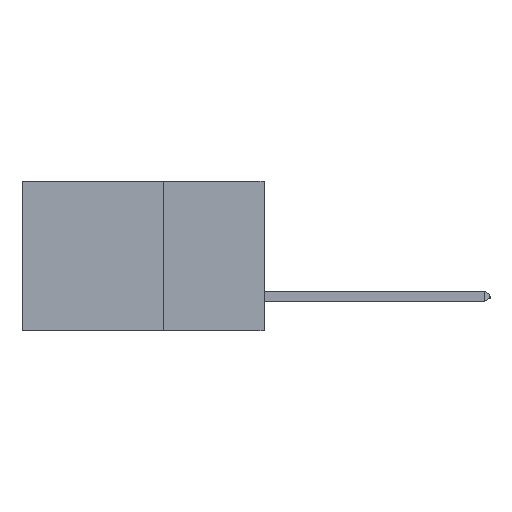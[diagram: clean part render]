
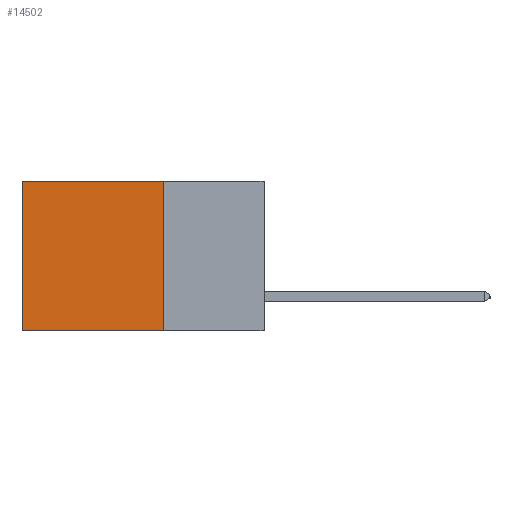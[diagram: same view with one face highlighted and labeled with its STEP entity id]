
A CAD part, left-side view. The second image highlights one B-rep face of the part: STEP entity #14502.
In plain terms, the highlighted planar face has unit normal (-1, 0, 0).
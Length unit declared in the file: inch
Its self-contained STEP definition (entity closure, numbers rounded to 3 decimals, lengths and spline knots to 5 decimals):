
#155 = VERTEX_POINT ( 'NONE', #8621 ) ;
#342 = DIRECTION ( 'NONE',  ( 1., 0., 0. ) ) ;
#1498 = EDGE_CURVE ( 'NONE', #5361, #14512, #9175, .T. ) ;
#1779 = LINE ( 'NONE', #20753, #18377 ) ;
#1804 = EDGE_CURVE ( 'NONE', #155, #20063, #20528, .T. ) ;
#2124 = EDGE_CURVE ( 'NONE', #155, #5361, #1779, .T. ) ;
#2147 = CARTESIAN_POINT ( 'NONE',  ( 0.298, 0.6, 0. ) ) ;
#3472 = CARTESIAN_POINT ( 'NONE',  ( 0.298, 0.25, 0. ) ) ;
#3716 = CARTESIAN_POINT ( 'NONE',  ( 0.298, 0.6, -0.37 ) ) ;
#5361 = VERTEX_POINT ( 'NONE', #2147 ) ;
#5472 = CARTESIAN_POINT ( 'NONE',  ( 0.298, 0.25, -0.37 ) ) ;
#5813 = CARTESIAN_POINT ( 'NONE',  ( 0.298, 0.25, -0.37 ) ) ;
#7941 = VECTOR ( 'NONE', #16961, 39.37008 ) ;
#8621 = CARTESIAN_POINT ( 'NONE',  ( 0.298, 0.25, 0. ) ) ;
#8667 = EDGE_LOOP ( 'NONE', ( #19448, #11887, #20361, #13693 ) ) ;
#9022 = DIRECTION ( 'NONE',  ( 0., 1., 0. ) ) ;
#9175 = LINE ( 'NONE', #17625, #14019 ) ;
#9632 = DIRECTION ( 'NONE',  ( 0., 0., -1. ) ) ;
#10149 = CARTESIAN_POINT ( 'NONE',  ( 0.298, 0.25, 0. ) ) ;
#10602 = FACE_OUTER_BOUND ( 'NONE', #8667, .T. ) ;
#11568 = EDGE_CURVE ( 'NONE', #20063, #14512, #12206, .T. ) ;
#11770 = DIRECTION ( 'NONE',  ( 0., 0., -1. ) ) ;
#11887 = ORIENTED_EDGE ( 'NONE', *, *, #11568, .F. ) ;
#12206 = LINE ( 'NONE', #5813, #20047 ) ;
#13693 = ORIENTED_EDGE ( 'NONE', *, *, #2124, .T. ) ;
#14019 = VECTOR ( 'NONE', #9632, 39.37008 ) ;
#14502 = ADVANCED_FACE ( 'NONE', ( #10602 ), #19624, .F. ) ;
#14512 = VERTEX_POINT ( 'NONE', #3716 ) ;
#16961 = DIRECTION ( 'NONE',  ( 0., 0., -1. ) ) ;
#17625 = CARTESIAN_POINT ( 'NONE',  ( 0.298, 0.6, 0. ) ) ;
#18377 = VECTOR ( 'NONE', #20114, 39.37008 ) ;
#19448 = ORIENTED_EDGE ( 'NONE', *, *, #1498, .T. ) ;
#19624 = PLANE ( 'NONE',  #19687 ) ;
#19687 = AXIS2_PLACEMENT_3D ( 'NONE', #10149, #342, #11770 ) ;
#20047 = VECTOR ( 'NONE', #9022, 39.37008 ) ;
#20063 = VERTEX_POINT ( 'NONE', #5472 ) ;
#20114 = DIRECTION ( 'NONE',  ( 0., 1., 0. ) ) ;
#20361 = ORIENTED_EDGE ( 'NONE', *, *, #1804, .F. ) ;
#20528 = LINE ( 'NONE', #3472, #7941 ) ;
#20753 = CARTESIAN_POINT ( 'NONE',  ( 0.298, 0.25, 0. ) ) ;
